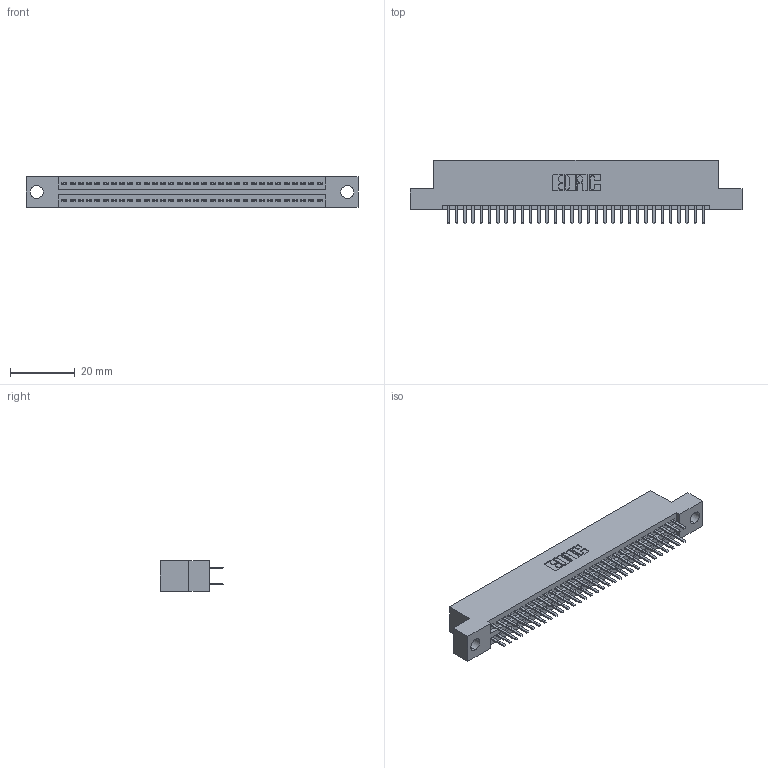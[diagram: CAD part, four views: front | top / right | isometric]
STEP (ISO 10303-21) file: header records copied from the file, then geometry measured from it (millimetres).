
FILE_DESCRIPTION (( 'STEP AP203' ), '1' );
FILE_NAME ('395-064-520-204.STEP', '2021-06-17T02:48:41', ( '' ), ( '' ), 'SwSTEP 2.0', 'SolidWorks 2020', '' );
FILE_SCHEMA (( 'CONFIG_CONTROL_DESIGN' ));
Length unit declared in the file: inch
Products named in the file (3): 345-292-001_345-293-120; 395-064-520-204; 345 Part_Flush Mounting Lugs - 0.156 Dia-TI
Assembly tree (65 placements, depth 2):
  395-064-520-204
    345 Part_Flush Mounting Lugs - 0.156 Dia-TI
    345-292-001_345-293-120  x64
Bounding box: 102.49 x 19.68 x 9.4 mm (x, y, z)
Volume: 9729 mm3; surface area: 13979.1 mm2
Topology: 65 solids, 65 shells, 3596 faces, 10425 edges, 6778 vertices
Faces by surface type: plane 2334, cylinder 1262
Entity records: 26987 total; most frequent: CARTESIAN_POINT 4550, ORIENTED_EDGE 4470, DIRECTION 4011, EDGE_CURVE 2235, VECTOR 1971, LINE 1971, VERTEX_POINT 1486, AXIS2_PLACEMENT_3D 1020
